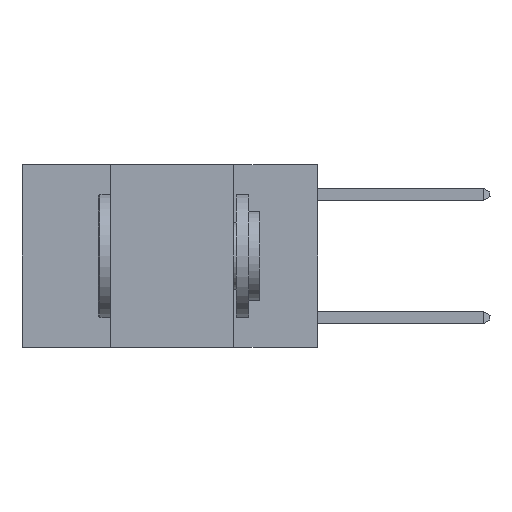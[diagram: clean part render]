
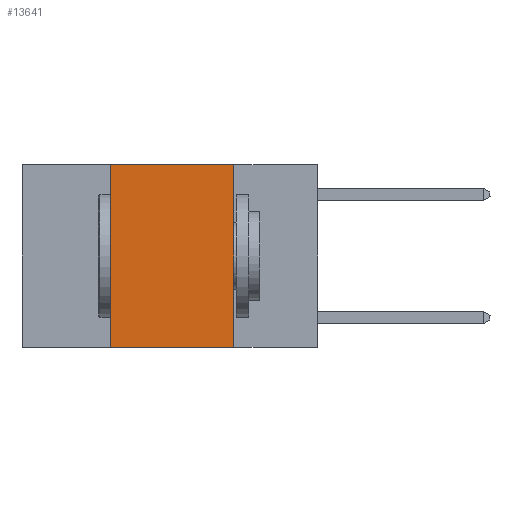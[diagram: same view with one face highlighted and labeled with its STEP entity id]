
A CAD part, left-side view. The second image highlights one B-rep face of the part: STEP entity #13641.
In plain terms, the highlighted planar face has unit normal (-1, 0, 0).
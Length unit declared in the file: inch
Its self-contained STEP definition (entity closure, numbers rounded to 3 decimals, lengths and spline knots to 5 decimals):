
#309 = FACE_OUTER_BOUND ( 'NONE', #14060, .T. ) ;
#1253 = EDGE_CURVE ( 'NONE', #3237, #28448, #5693, .T. ) ;
#1728 = VERTEX_POINT ( 'NONE', #27390 ) ;
#1806 = DIRECTION ( 'NONE',  ( 0., 0., -1. ) ) ;
#3199 = PLANE ( 'NONE',  #6689 ) ;
#3237 = VERTEX_POINT ( 'NONE', #22732 ) ;
#3861 = LINE ( 'NONE', #7080, #21869 ) ;
#4719 = LINE ( 'NONE', #8763, #28833 ) ;
#5693 = LINE ( 'NONE', #26779, #29071 ) ;
#6689 = AXIS2_PLACEMENT_3D ( 'NONE', #12708, #28967, #15094 ) ;
#7080 = CARTESIAN_POINT ( 'NONE',  ( 0., 0.42, 0. ) ) ;
#7755 = EDGE_CURVE ( 'NONE', #16947, #1728, #17941, .T. ) ;
#8763 = CARTESIAN_POINT ( 'NONE',  ( 0., 0.17, 0. ) ) ;
#10939 = VECTOR ( 'NONE', #11400, 39.37008 ) ;
#11400 = DIRECTION ( 'NONE',  ( 0., -1., 0. ) ) ;
#12708 = CARTESIAN_POINT ( 'NONE',  ( 0., 0.6, 0. ) ) ;
#13641 = ADVANCED_FACE ( 'NONE', ( #309 ), #3199, .F. ) ;
#14060 = EDGE_LOOP ( 'NONE', ( #14738, #14848, #15595, #15655 ) ) ;
#14738 = ORIENTED_EDGE ( 'NONE', *, *, #19782, .F. ) ;
#14848 = ORIENTED_EDGE ( 'NONE', *, *, #1253, .F. ) ;
#15094 = DIRECTION ( 'NONE',  ( 0., 0., -1. ) ) ;
#15595 = ORIENTED_EDGE ( 'NONE', *, *, #16293, .F. ) ;
#15655 = ORIENTED_EDGE ( 'NONE', *, *, #7755, .T. ) ;
#16293 = EDGE_CURVE ( 'NONE', #16947, #3237, #3861, .T. ) ;
#16947 = VERTEX_POINT ( 'NONE', #23220 ) ;
#17941 = LINE ( 'NONE', #23008, #10939 ) ;
#18487 = DIRECTION ( 'NONE',  ( 0., -1., 0. ) ) ;
#19777 = CARTESIAN_POINT ( 'NONE',  ( 0., 0.17, 0. ) ) ;
#19782 = EDGE_CURVE ( 'NONE', #28448, #1728, #4719, .T. ) ;
#21139 = DIRECTION ( 'NONE',  ( 0., 0., 1. ) ) ;
#21869 = VECTOR ( 'NONE', #21139, 39.37008 ) ;
#22732 = CARTESIAN_POINT ( 'NONE',  ( 0., 0.42, 0. ) ) ;
#23008 = CARTESIAN_POINT ( 'NONE',  ( 0., 0.6, -0.37 ) ) ;
#23220 = CARTESIAN_POINT ( 'NONE',  ( 0., 0.42, -0.37 ) ) ;
#26779 = CARTESIAN_POINT ( 'NONE',  ( 0., 0.6, 0. ) ) ;
#27390 = CARTESIAN_POINT ( 'NONE',  ( 0., 0.17, -0.37 ) ) ;
#28448 = VERTEX_POINT ( 'NONE', #19777 ) ;
#28833 = VECTOR ( 'NONE', #1806, 39.37008 ) ;
#28967 = DIRECTION ( 'NONE',  ( 1., 0., 0. ) ) ;
#29071 = VECTOR ( 'NONE', #18487, 39.37008 ) ;
